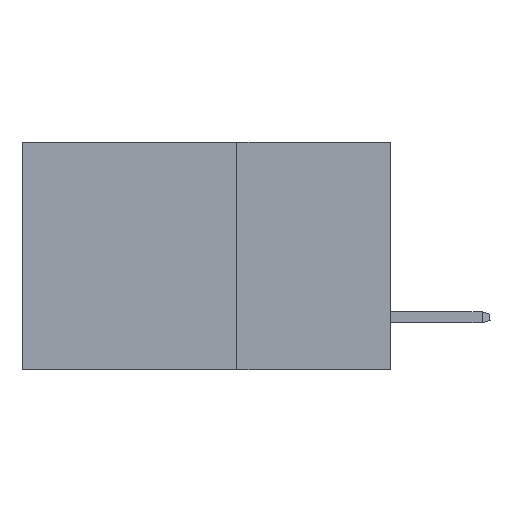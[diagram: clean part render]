
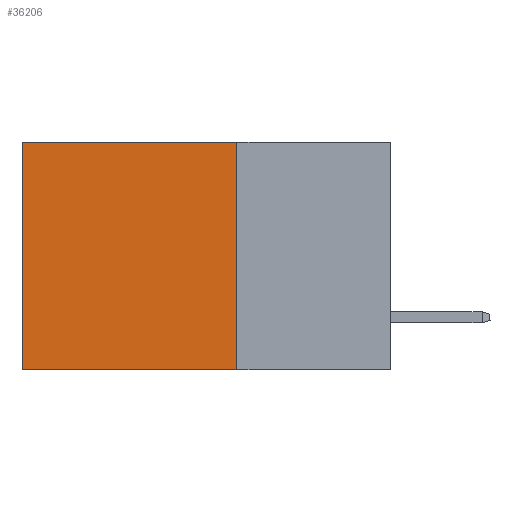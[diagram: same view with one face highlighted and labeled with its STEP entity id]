
A CAD part, left-side view. The second image highlights one B-rep face of the part: STEP entity #36206.
In plain terms, the highlighted planar face has unit normal (-1, 0, 0).
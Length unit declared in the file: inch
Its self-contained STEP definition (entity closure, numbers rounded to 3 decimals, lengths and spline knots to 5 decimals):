
#1408 = CARTESIAN_POINT ( 'NONE',  ( 0.2875, 0.25, 0. ) ) ;
#1507 = FACE_OUTER_BOUND ( 'NONE', #42461, .T. ) ;
#2084 = EDGE_CURVE ( 'NONE', #22071, #10626, #38275, .T. ) ;
#2872 = VERTEX_POINT ( 'NONE', #3617 ) ;
#3617 = CARTESIAN_POINT ( 'NONE',  ( 0.2875, 0.25, -0.37 ) ) ;
#4115 = CARTESIAN_POINT ( 'NONE',  ( 0.2875, 0.6, -0.37 ) ) ;
#6441 = LINE ( 'NONE', #45937, #44368 ) ;
#7284 = LINE ( 'NONE', #17523, #13615 ) ;
#7531 = AXIS2_PLACEMENT_3D ( 'NONE', #1408, #32785, #24738 ) ;
#7587 = CARTESIAN_POINT ( 'NONE',  ( 0.2875, 0.6, 0. ) ) ;
#8787 = PLANE ( 'NONE',  #7531 ) ;
#10626 = VERTEX_POINT ( 'NONE', #28614 ) ;
#11833 = ORIENTED_EDGE ( 'NONE', *, *, #39257, .F. ) ;
#12021 = DIRECTION ( 'NONE',  ( 0., 0., -1. ) ) ;
#13243 = EDGE_CURVE ( 'NONE', #10626, #46866, #39544, .T. ) ;
#13615 = VECTOR ( 'NONE', #28871, 39.37008 ) ;
#14281 = CARTESIAN_POINT ( 'NONE',  ( 0.2875, 0.25, 0. ) ) ;
#17523 = CARTESIAN_POINT ( 'NONE',  ( 0.2875, 0.25, -0.37 ) ) ;
#22071 = VERTEX_POINT ( 'NONE', #36058 ) ;
#23599 = DIRECTION ( 'NONE',  ( 0., 0., -1. ) ) ;
#23665 = VECTOR ( 'NONE', #30310, 39.37008 ) ;
#24254 = ORIENTED_EDGE ( 'NONE', *, *, #13243, .T. ) ;
#24738 = DIRECTION ( 'NONE',  ( 0., 0., -1. ) ) ;
#28614 = CARTESIAN_POINT ( 'NONE',  ( 0.2875, 0.6, 0. ) ) ;
#28717 = EDGE_CURVE ( 'NONE', #2872, #46866, #7284, .T. ) ;
#28871 = DIRECTION ( 'NONE',  ( 0., 1., 0. ) ) ;
#29685 = VECTOR ( 'NONE', #12021, 39.37008 ) ;
#30310 = DIRECTION ( 'NONE',  ( 0., 1., 0. ) ) ;
#32785 = DIRECTION ( 'NONE',  ( 1., 0., 0. ) ) ;
#35256 = ORIENTED_EDGE ( 'NONE', *, *, #28717, .F. ) ;
#36058 = CARTESIAN_POINT ( 'NONE',  ( 0.2875, 0.25, 0. ) ) ;
#36206 = ADVANCED_FACE ( 'NONE', ( #1507 ), #8787, .F. ) ;
#38275 = LINE ( 'NONE', #14281, #23665 ) ;
#39257 = EDGE_CURVE ( 'NONE', #22071, #2872, #6441, .T. ) ;
#39544 = LINE ( 'NONE', #7587, #29685 ) ;
#42461 = EDGE_LOOP ( 'NONE', ( #24254, #35256, #11833, #48029 ) ) ;
#44368 = VECTOR ( 'NONE', #23599, 39.37008 ) ;
#45937 = CARTESIAN_POINT ( 'NONE',  ( 0.2875, 0.25, 0. ) ) ;
#46866 = VERTEX_POINT ( 'NONE', #4115 ) ;
#48029 = ORIENTED_EDGE ( 'NONE', *, *, #2084, .T. ) ;
